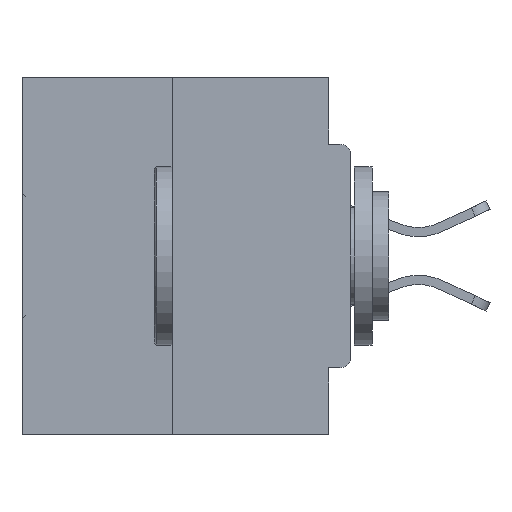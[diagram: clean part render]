
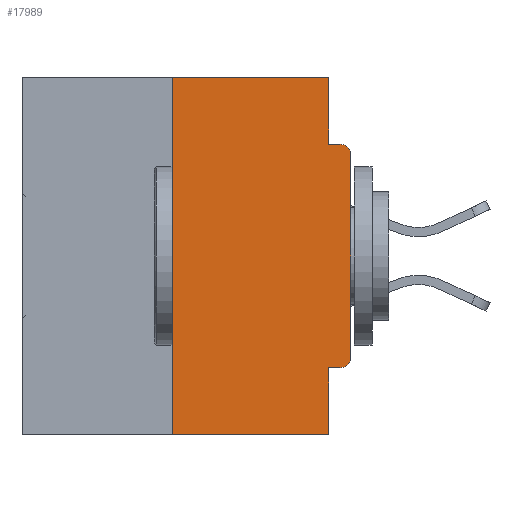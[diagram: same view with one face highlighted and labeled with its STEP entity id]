
A CAD part, left-side view. The second image highlights one B-rep face of the part: STEP entity #17989.
In plain terms, the highlighted planar face has unit normal (-1, 0, 0).
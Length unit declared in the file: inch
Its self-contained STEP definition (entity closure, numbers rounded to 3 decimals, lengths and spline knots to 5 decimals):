
#271 = VERTEX_POINT ( 'NONE', #39049 ) ;
#733 = CARTESIAN_POINT ( 'NONE',  ( 0., 0., -0.4065 ) ) ;
#1236 = EDGE_CURVE ( 'NONE', #13516, #5050, #13177, .T. ) ;
#1320 = DIRECTION ( 'NONE',  ( -1., 0., 0. ) ) ;
#1473 = LINE ( 'NONE', #32585, #9233 ) ;
#2881 = ORIENTED_EDGE ( 'NONE', *, *, #32173, .F. ) ;
#3883 = DIRECTION ( 'NONE',  ( 0., 0., -1. ) ) ;
#4877 = DIRECTION ( 'NONE',  ( 0., 0., -1. ) ) ;
#5049 = DIRECTION ( 'NONE',  ( 0., -1., 0. ) ) ;
#5050 = VERTEX_POINT ( 'NONE', #13737 ) ;
#5597 = LINE ( 'NONE', #733, #13327 ) ;
#7557 = ORIENTED_EDGE ( 'NONE', *, *, #36958, .T. ) ;
#7800 = LINE ( 'NONE', #19210, #27923 ) ;
#8215 = VECTOR ( 'NONE', #5049, 39.37008 ) ;
#8262 = DIRECTION ( 'NONE',  ( 0., 0., -1. ) ) ;
#9233 = VECTOR ( 'NONE', #35916, 39.37008 ) ;
#9409 = LINE ( 'NONE', #40689, #24921 ) ;
#9824 = EDGE_CURVE ( 'NONE', #5050, #41627, #1473, .T. ) ;
#10099 = CARTESIAN_POINT ( 'NONE',  ( 0., 0., 0. ) ) ;
#10669 = CARTESIAN_POINT ( 'NONE',  ( 0., 0.46, 0. ) ) ;
#13177 = LINE ( 'NONE', #40562, #41722 ) ;
#13327 = VECTOR ( 'NONE', #24138, 39.37008 ) ;
#13516 = VERTEX_POINT ( 'NONE', #39611 ) ;
#13737 = CARTESIAN_POINT ( 'NONE',  ( 0., 0.25, 0. ) ) ;
#14495 = ORIENTED_EDGE ( 'NONE', *, *, #25525, .T. ) ;
#14765 = ORIENTED_EDGE ( 'NONE', *, *, #38494, .T. ) ;
#15178 = DIRECTION ( 'NONE',  ( 0., 0., -1. ) ) ;
#15248 = VERTEX_POINT ( 'NONE', #37090 ) ;
#15646 = FACE_OUTER_BOUND ( 'NONE', #17005, .T. ) ;
#16011 = VERTEX_POINT ( 'NONE', #26564 ) ;
#17005 = EDGE_LOOP ( 'NONE', ( #29813, #36598, #14495, #29642, #35007, #7557, #41800, #14765, #40724, #2881 ) ) ;
#17989 = ADVANCED_FACE ( 'NONE', ( #15646 ), #30486, .F. ) ;
#18902 = CARTESIAN_POINT ( 'NONE',  ( 0., 0.031, 0. ) ) ;
#19072 = VERTEX_POINT ( 'NONE', #20503 ) ;
#19210 = CARTESIAN_POINT ( 'NONE',  ( 0., 0.46, -0.5 ) ) ;
#20092 = DIRECTION ( 'NONE',  ( 0., 0., 1. ) ) ;
#20503 = CARTESIAN_POINT ( 'NONE',  ( 0., 0.015, -0.0935 ) ) ;
#21102 = CARTESIAN_POINT ( 'NONE',  ( 0., 0.031, 0. ) ) ;
#21107 = VECTOR ( 'NONE', #15178, 39.37008 ) ;
#21309 = EDGE_CURVE ( 'NONE', #38636, #15248, #9409, .T. ) ;
#21389 = DIRECTION ( 'NONE',  ( 0., 0., -1. ) ) ;
#22293 = AXIS2_PLACEMENT_3D ( 'NONE', #41264, #1320, #8262 ) ;
#23136 = LINE ( 'NONE', #18902, #21107 ) ;
#23499 = CARTESIAN_POINT ( 'NONE',  ( 0., 0.031, -0.4065 ) ) ;
#23608 = CIRCLE ( 'NONE', #22293, 0.015 ) ;
#24138 = DIRECTION ( 'NONE',  ( 0., 1., 0. ) ) ;
#24921 = VECTOR ( 'NONE', #21389, 39.37008 ) ;
#25525 = EDGE_CURVE ( 'NONE', #13516, #15248, #7800, .T. ) ;
#26081 = EDGE_CURVE ( 'NONE', #30991, #26652, #41385, .T. ) ;
#26564 = CARTESIAN_POINT ( 'NONE',  ( 0., 0.031, -0.0935 ) ) ;
#26652 = VERTEX_POINT ( 'NONE', #37364 ) ;
#26801 = AXIS2_PLACEMENT_3D ( 'NONE', #10669, #34659, #4877 ) ;
#26805 = LINE ( 'NONE', #27624, #8215 ) ;
#27624 = CARTESIAN_POINT ( 'NONE',  ( 0., 0., -0.0935 ) ) ;
#27923 = VECTOR ( 'NONE', #29317, 39.37008 ) ;
#29317 = DIRECTION ( 'NONE',  ( 0., -1., 0. ) ) ;
#29642 = ORIENTED_EDGE ( 'NONE', *, *, #21309, .F. ) ;
#29813 = ORIENTED_EDGE ( 'NONE', *, *, #9824, .F. ) ;
#30157 = CIRCLE ( 'NONE', #36743, 0.015 ) ;
#30486 = PLANE ( 'NONE',  #26801 ) ;
#30930 = CARTESIAN_POINT ( 'NONE',  ( 0., 0.015, -0.1085 ) ) ;
#30991 = VERTEX_POINT ( 'NONE', #33469 ) ;
#31493 = VECTOR ( 'NONE', #20092, 39.37008 ) ;
#31918 = EDGE_CURVE ( 'NONE', #271, #38636, #5597, .T. ) ;
#31978 = EDGE_CURVE ( 'NONE', #16011, #19072, #26805, .T. ) ;
#32173 = EDGE_CURVE ( 'NONE', #41627, #16011, #23136, .T. ) ;
#32585 = CARTESIAN_POINT ( 'NONE',  ( 0., 0.46, 0. ) ) ;
#33469 = CARTESIAN_POINT ( 'NONE',  ( 0., 0., -0.3915 ) ) ;
#34659 = DIRECTION ( 'NONE',  ( 1., 0., 0. ) ) ;
#35007 = ORIENTED_EDGE ( 'NONE', *, *, #31918, .F. ) ;
#35916 = DIRECTION ( 'NONE',  ( 0., -1., 0. ) ) ;
#36598 = ORIENTED_EDGE ( 'NONE', *, *, #1236, .F. ) ;
#36743 = AXIS2_PLACEMENT_3D ( 'NONE', #30930, #40187, #3883 ) ;
#36958 = EDGE_CURVE ( 'NONE', #271, #30991, #23608, .T. ) ;
#37090 = CARTESIAN_POINT ( 'NONE',  ( 0., 0.031, -0.5 ) ) ;
#37364 = CARTESIAN_POINT ( 'NONE',  ( 0., 0., -0.1085 ) ) ;
#37609 = DIRECTION ( 'NONE',  ( 0., 0., 1. ) ) ;
#38494 = EDGE_CURVE ( 'NONE', #26652, #19072, #30157, .T. ) ;
#38636 = VERTEX_POINT ( 'NONE', #23499 ) ;
#39049 = CARTESIAN_POINT ( 'NONE',  ( 0., 0.015, -0.4065 ) ) ;
#39611 = CARTESIAN_POINT ( 'NONE',  ( 0., 0.25, -0.5 ) ) ;
#40187 = DIRECTION ( 'NONE',  ( -1., 0., 0. ) ) ;
#40562 = CARTESIAN_POINT ( 'NONE',  ( 0., 0.25, 0. ) ) ;
#40689 = CARTESIAN_POINT ( 'NONE',  ( 0., 0.031, -0.5 ) ) ;
#40724 = ORIENTED_EDGE ( 'NONE', *, *, #31978, .F. ) ;
#41264 = CARTESIAN_POINT ( 'NONE',  ( 0., 0.015, -0.3915 ) ) ;
#41385 = LINE ( 'NONE', #10099, #31493 ) ;
#41627 = VERTEX_POINT ( 'NONE', #21102 ) ;
#41722 = VECTOR ( 'NONE', #37609, 39.37008 ) ;
#41800 = ORIENTED_EDGE ( 'NONE', *, *, #26081, .T. ) ;
